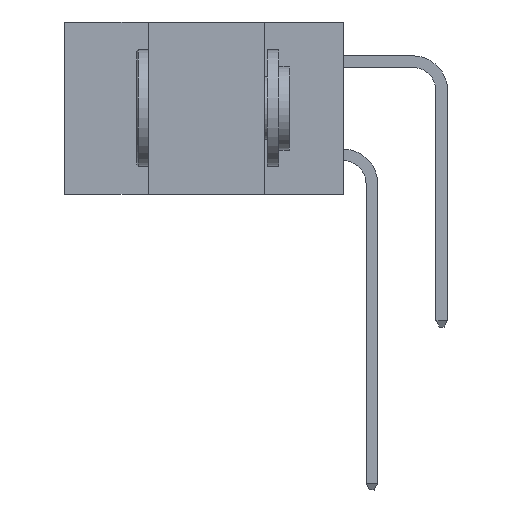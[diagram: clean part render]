
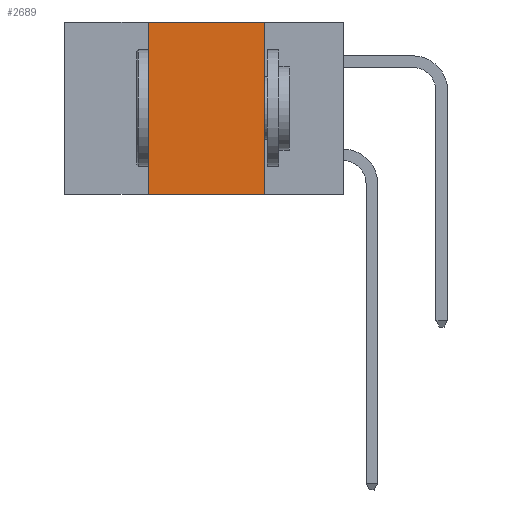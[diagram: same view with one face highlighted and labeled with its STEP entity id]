
A CAD part, left-side view. The second image highlights one B-rep face of the part: STEP entity #2689.
In plain terms, the highlighted planar face has unit normal (-1, 0, 0).
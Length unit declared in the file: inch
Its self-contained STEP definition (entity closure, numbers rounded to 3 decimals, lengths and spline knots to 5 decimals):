
#161 = CARTESIAN_POINT ( 'NONE',  ( 0., 0.6, -0.37 ) ) ;
#463 = CARTESIAN_POINT ( 'NONE',  ( 0., 0.42, 0. ) ) ;
#598 = VECTOR ( 'NONE', #3057, 39.37008 ) ;
#2197 = VECTOR ( 'NONE', #11381, 39.37008 ) ;
#2219 = EDGE_CURVE ( 'NONE', #9707, #12898, #6450, .T. ) ;
#2689 = ADVANCED_FACE ( 'NONE', ( #14127 ), #8980, .F. ) ;
#3057 = DIRECTION ( 'NONE',  ( 0., 0., -1. ) ) ;
#3579 = LINE ( 'NONE', #11988, #598 ) ;
#3791 = DIRECTION ( 'NONE',  ( 0., -1., 0. ) ) ;
#4007 = VECTOR ( 'NONE', #8168, 39.37008 ) ;
#4254 = EDGE_CURVE ( 'NONE', #12898, #5926, #7076, .T. ) ;
#4436 = CARTESIAN_POINT ( 'NONE',  ( 0., 0.6, 0. ) ) ;
#4526 = CARTESIAN_POINT ( 'NONE',  ( 0., 0.17, -0.37 ) ) ;
#4538 = DIRECTION ( 'NONE',  ( 1., 0., 0. ) ) ;
#4577 = EDGE_CURVE ( 'NONE', #5926, #8497, #3579, .T. ) ;
#5090 = CARTESIAN_POINT ( 'NONE',  ( 0., 0.42, 0. ) ) ;
#5926 = VERTEX_POINT ( 'NONE', #14430 ) ;
#6450 = LINE ( 'NONE', #463, #4007 ) ;
#7045 = VECTOR ( 'NONE', #3791, 39.37008 ) ;
#7076 = LINE ( 'NONE', #11481, #2197 ) ;
#7890 = LINE ( 'NONE', #161, #7045 ) ;
#8168 = DIRECTION ( 'NONE',  ( 0., 0., 1. ) ) ;
#8497 = VERTEX_POINT ( 'NONE', #4526 ) ;
#8868 = AXIS2_PLACEMENT_3D ( 'NONE', #4436, #4538, #13471 ) ;
#8980 = PLANE ( 'NONE',  #8868 ) ;
#9318 = EDGE_CURVE ( 'NONE', #9707, #8497, #7890, .T. ) ;
#9707 = VERTEX_POINT ( 'NONE', #10757 ) ;
#9721 = EDGE_LOOP ( 'NONE', ( #10680, #13204, #11456, #10899 ) ) ;
#10680 = ORIENTED_EDGE ( 'NONE', *, *, #4577, .F. ) ;
#10757 = CARTESIAN_POINT ( 'NONE',  ( 0., 0.42, -0.37 ) ) ;
#10899 = ORIENTED_EDGE ( 'NONE', *, *, #9318, .T. ) ;
#11381 = DIRECTION ( 'NONE',  ( 0., -1., 0. ) ) ;
#11456 = ORIENTED_EDGE ( 'NONE', *, *, #2219, .F. ) ;
#11481 = CARTESIAN_POINT ( 'NONE',  ( 0., 0.6, 0. ) ) ;
#11988 = CARTESIAN_POINT ( 'NONE',  ( 0., 0.17, 0. ) ) ;
#12898 = VERTEX_POINT ( 'NONE', #5090 ) ;
#13204 = ORIENTED_EDGE ( 'NONE', *, *, #4254, .F. ) ;
#13471 = DIRECTION ( 'NONE',  ( 0., 0., -1. ) ) ;
#14127 = FACE_OUTER_BOUND ( 'NONE', #9721, .T. ) ;
#14430 = CARTESIAN_POINT ( 'NONE',  ( 0., 0.17, 0. ) ) ;
